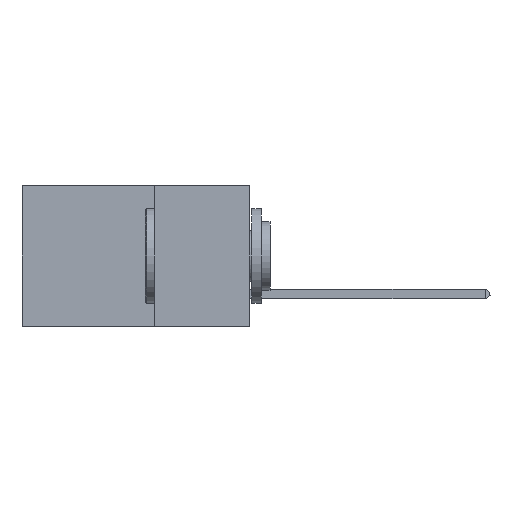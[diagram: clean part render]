
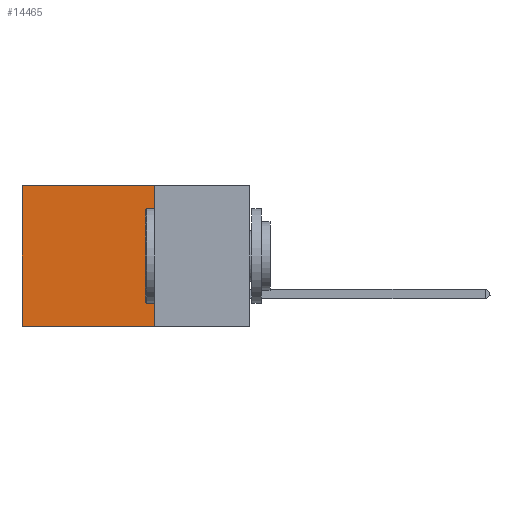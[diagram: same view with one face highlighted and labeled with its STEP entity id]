
A CAD part, left-side view. The second image highlights one B-rep face of the part: STEP entity #14465.
In plain terms, the highlighted planar face has unit normal (-1, 0, 0).
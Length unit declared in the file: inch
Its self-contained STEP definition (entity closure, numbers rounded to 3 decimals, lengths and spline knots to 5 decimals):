
#815 = VECTOR ( 'NONE', #14852, 39.37008 ) ;
#1333 = ORIENTED_EDGE ( 'NONE', *, *, #10320, .T. ) ;
#1869 = LINE ( 'NONE', #15383, #12529 ) ;
#1975 = EDGE_CURVE ( 'NONE', #10221, #14340, #1869, .T. ) ;
#3295 = ORIENTED_EDGE ( 'NONE', *, *, #1975, .T. ) ;
#3394 = CARTESIAN_POINT ( 'NONE',  ( 0.2875, 0.25, -0.37 ) ) ;
#3624 = EDGE_CURVE ( 'NONE', #8725, #5489, #6822, .T. ) ;
#4160 = DIRECTION ( 'NONE',  ( 1., 0., 0. ) ) ;
#4344 = CARTESIAN_POINT ( 'NONE',  ( 0.2875, 0.25, 0. ) ) ;
#4894 = VECTOR ( 'NONE', #14558, 39.37008 ) ;
#4962 = LINE ( 'NONE', #12065, #815 ) ;
#5049 = DIRECTION ( 'NONE',  ( 0., 0., -1. ) ) ;
#5489 = VERTEX_POINT ( 'NONE', #14670 ) ;
#5551 = CARTESIAN_POINT ( 'NONE',  ( 0.2875, 0.25, 0. ) ) ;
#5756 = EDGE_LOOP ( 'NONE', ( #3295, #13897, #13779, #1333 ) ) ;
#6106 = CARTESIAN_POINT ( 'NONE',  ( 0.2875, 0.6, -0.37 ) ) ;
#6474 = CARTESIAN_POINT ( 'NONE',  ( 0.2875, 0.6, 0. ) ) ;
#6822 = LINE ( 'NONE', #11977, #13996 ) ;
#7446 = AXIS2_PLACEMENT_3D ( 'NONE', #4344, #4160, #12467 ) ;
#8725 = VERTEX_POINT ( 'NONE', #5551 ) ;
#9540 = FACE_OUTER_BOUND ( 'NONE', #5756, .T. ) ;
#10221 = VERTEX_POINT ( 'NONE', #6474 ) ;
#10320 = EDGE_CURVE ( 'NONE', #8725, #10221, #4962, .T. ) ;
#11889 = EDGE_CURVE ( 'NONE', #5489, #14340, #16885, .T. ) ;
#11977 = CARTESIAN_POINT ( 'NONE',  ( 0.2875, 0.25, 0. ) ) ;
#12065 = CARTESIAN_POINT ( 'NONE',  ( 0.2875, 0.25, 0. ) ) ;
#12467 = DIRECTION ( 'NONE',  ( 0., 0., -1. ) ) ;
#12526 = PLANE ( 'NONE',  #7446 ) ;
#12529 = VECTOR ( 'NONE', #13898, 39.37008 ) ;
#13779 = ORIENTED_EDGE ( 'NONE', *, *, #3624, .F. ) ;
#13897 = ORIENTED_EDGE ( 'NONE', *, *, #11889, .F. ) ;
#13898 = DIRECTION ( 'NONE',  ( 0., 0., -1. ) ) ;
#13996 = VECTOR ( 'NONE', #5049, 39.37008 ) ;
#14340 = VERTEX_POINT ( 'NONE', #6106 ) ;
#14465 = ADVANCED_FACE ( 'NONE', ( #9540 ), #12526, .F. ) ;
#14558 = DIRECTION ( 'NONE',  ( 0., 1., 0. ) ) ;
#14670 = CARTESIAN_POINT ( 'NONE',  ( 0.2875, 0.25, -0.37 ) ) ;
#14852 = DIRECTION ( 'NONE',  ( 0., 1., 0. ) ) ;
#15383 = CARTESIAN_POINT ( 'NONE',  ( 0.2875, 0.6, 0. ) ) ;
#16885 = LINE ( 'NONE', #3394, #4894 ) ;
